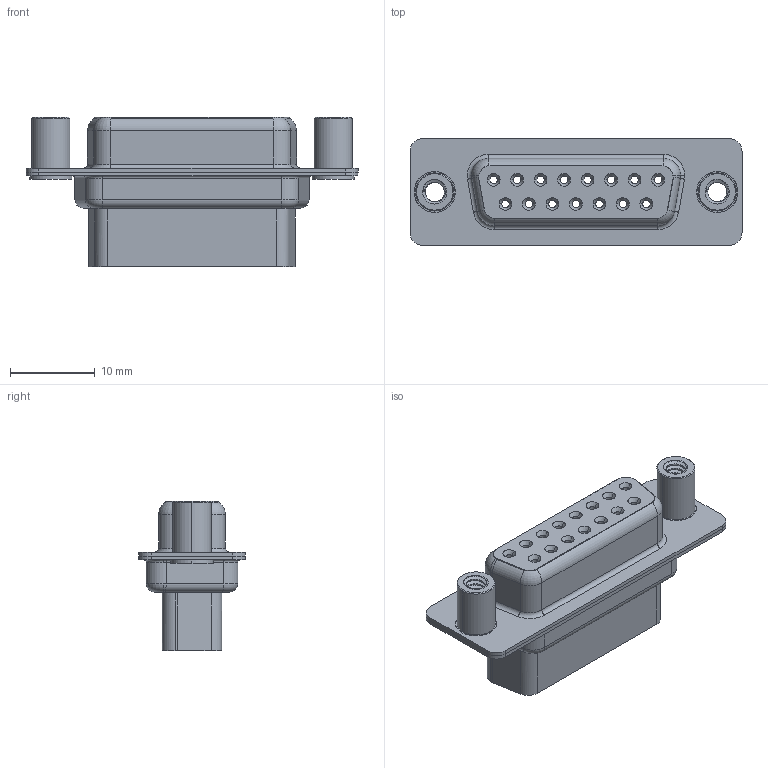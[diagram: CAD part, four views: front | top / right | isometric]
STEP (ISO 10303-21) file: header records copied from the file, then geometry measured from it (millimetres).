
FILE_DESCRIPTION (( 'STEP AP203' ), '1' );
FILE_NAME ('628-015-010-041.STEP', '2020-07-15T20:23:31', ( '' ), ( '' ), 'SwSTEP 2.0', 'SolidWorks 2020', '' );
FILE_SCHEMA (( 'CONFIG_CONTROL_DESIGN' ));
Length unit declared in the file: millimetre
Products named in the file (5): 628 4-40 Threaded Standoff; 628 Shell Front_15 Contacts; 628 Shell Rear_15 Contacts; 628-015-010-041; 628 Housing_15 HP
Assembly tree (5 placements, depth 2):
  628-015-010-041
    628 Housing_15 HP
    628 Shell Front_15 Contacts
    628 Shell Rear_15 Contacts
    628 4-40 Threaded Standoff  x2
Bounding box: 39.15 x 12.6 x 17.6 mm (x, y, z)
Volume: 3151.8 mm3; surface area: 5734.1 mm2
Topology: 5 solids, 5 shells, 508 faces, 1199 edges, 759 vertices
Faces by surface type: cylinder 285, plane 114, torus 63, cone 40, bspline 6
Entity records: 15552 total; most frequent: CARTESIAN_POINT 4185, DIRECTION 2451, ORIENTED_EDGE 2142, EDGE_CURVE 1071, AXIS2_PLACEMENT_3D 1020, VERTEX_POINT 676, EDGE_LOOP 557, CIRCLE 557
